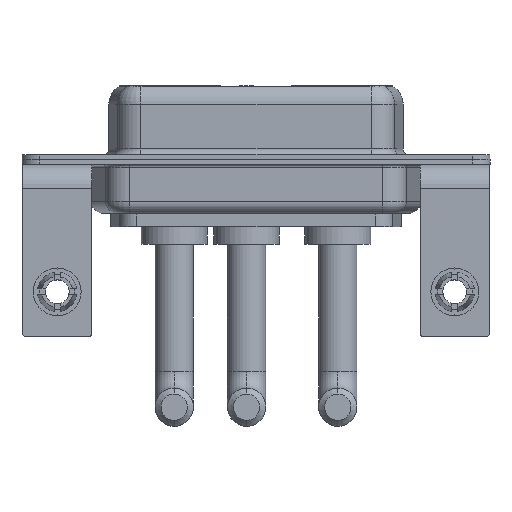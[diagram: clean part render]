
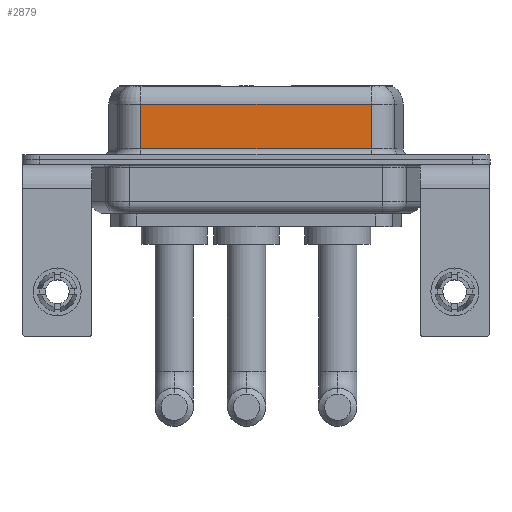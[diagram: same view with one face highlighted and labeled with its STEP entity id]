
A CAD part, front view. The second image highlights one B-rep face of the part: STEP entity #2879.
In plain terms, the highlighted planar face has unit normal (0, -1, 0).
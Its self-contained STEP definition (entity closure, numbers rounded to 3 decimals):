
#528 = ORIENTED_EDGE ( 'NONE', *, *, #4149, .T. ) ;
#1212 = VECTOR ( 'NONE', #8335, 1000. ) ;
#1411 = AXIS2_PLACEMENT_3D ( 'NONE', #6801, #9167, #11767 ) ;
#1601 = CARTESIAN_POINT ( 'NONE',  ( 7.013, -3.95, 0.9 ) ) ;
#2879 = ADVANCED_FACE ( 'NONE', ( #15377 ), #4203, .F. ) ;
#3974 = EDGE_LOOP ( 'NONE', ( #15123, #528, #10780, #15513 ) ) ;
#4142 = DIRECTION ( 'NONE',  ( 1., 0., 0. ) ) ;
#4149 = EDGE_CURVE ( 'NONE', #12173, #6477, #12291, .T. ) ;
#4203 = PLANE ( 'NONE',  #1411 ) ;
#4721 = CARTESIAN_POINT ( 'NONE',  ( 7.013, -3.95, 4.65 ) ) ;
#6048 = VECTOR ( 'NONE', #6171, 1000. ) ;
#6171 = DIRECTION ( 'NONE',  ( 0., 0., -1. ) ) ;
#6477 = VERTEX_POINT ( 'NONE', #4721 ) ;
#6705 = EDGE_CURVE ( 'NONE', #6477, #10146, #9275, .T. ) ;
#6801 = CARTESIAN_POINT ( 'NONE',  ( 26.287, -3.95, 6.4 ) ) ;
#6834 = CARTESIAN_POINT ( 'NONE',  ( 7.013, -3.95, 6.4 ) ) ;
#7264 = CARTESIAN_POINT ( 'NONE',  ( 26.287, -3.95, 4.65 ) ) ;
#8227 = EDGE_CURVE ( 'NONE', #10146, #8687, #14407, .T. ) ;
#8335 = DIRECTION ( 'NONE',  ( -1., 0., 0. ) ) ;
#8470 = LINE ( 'NONE', #14747, #6048 ) ;
#8687 = VERTEX_POINT ( 'NONE', #9090 ) ;
#9090 = CARTESIAN_POINT ( 'NONE',  ( 26.287, -3.95, 0.9 ) ) ;
#9167 = DIRECTION ( 'NONE',  ( 0., 1., 0. ) ) ;
#9189 = CARTESIAN_POINT ( 'NONE',  ( 26.287, -3.95, 0.9 ) ) ;
#9275 = LINE ( 'NONE', #6834, #15353 ) ;
#9977 = EDGE_CURVE ( 'NONE', #12173, #8687, #8470, .T. ) ;
#10146 = VERTEX_POINT ( 'NONE', #1601 ) ;
#10780 = ORIENTED_EDGE ( 'NONE', *, *, #6705, .T. ) ;
#11564 = DIRECTION ( 'NONE',  ( 0., 0., -1. ) ) ;
#11767 = DIRECTION ( 'NONE',  ( 0., 0., 1. ) ) ;
#12173 = VERTEX_POINT ( 'NONE', #14158 ) ;
#12291 = LINE ( 'NONE', #7264, #1212 ) ;
#14158 = CARTESIAN_POINT ( 'NONE',  ( 26.287, -3.95, 4.65 ) ) ;
#14338 = VECTOR ( 'NONE', #4142, 1000. ) ;
#14407 = LINE ( 'NONE', #9189, #14338 ) ;
#14747 = CARTESIAN_POINT ( 'NONE',  ( 26.287, -3.95, 6.4 ) ) ;
#15123 = ORIENTED_EDGE ( 'NONE', *, *, #9977, .F. ) ;
#15353 = VECTOR ( 'NONE', #11564, 1000. ) ;
#15377 = FACE_OUTER_BOUND ( 'NONE', #3974, .T. ) ;
#15513 = ORIENTED_EDGE ( 'NONE', *, *, #8227, .T. ) ;
